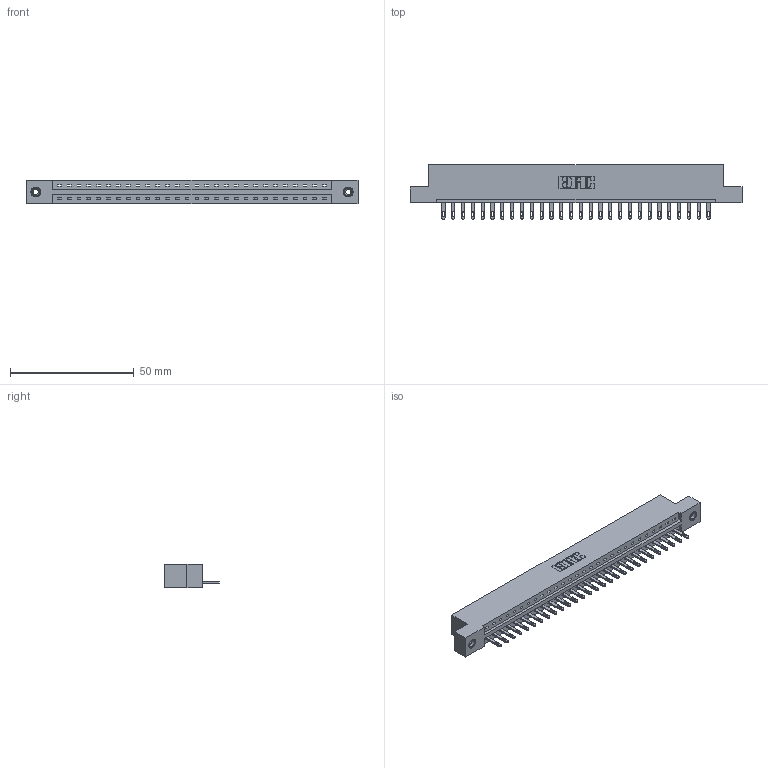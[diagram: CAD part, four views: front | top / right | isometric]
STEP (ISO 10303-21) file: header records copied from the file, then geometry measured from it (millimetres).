
FILE_DESCRIPTION (( 'STEP AP203' ), '1' );
FILE_NAME ('337-028-500-108.STEP', '2018-08-06T08:46:16', ( '' ), ( '' ), 'SwSTEP 2.0', 'SolidWorks 2016', '' );
FILE_SCHEMA (( 'CONFIG_CONTROL_DESIGN' ));
Length unit declared in the file: inch
Products named in the file (4): 337 Part_Flush Mounting Lugs - 0.156 Dia-TI; 345-292-001_345-293-100; 345-250-001_345-250-003-102; 337-028-500-108
Assembly tree (31 placements, depth 2):
  337-028-500-108
    337 Part_Flush Mounting Lugs - 0.156 Dia-TI
    345-292-001_345-293-100  x28
    345-250-001_345-250-003-102  x2
Bounding box: 133.96 x 21.85 x 9.4 mm (x, y, z)
Volume: 13758.5 mm3; surface area: 14234.7 mm2
Topology: 31 solids, 31 shells, 1798 faces, 5487 edges, 3650 vertices
Faces by surface type: plane 1222, cylinder 560, cone 12, torus 4
Entity records: 23740 total; most frequent: CARTESIAN_POINT 4113, ORIENTED_EDGE 4070, DIRECTION 3525, EDGE_CURVE 2035, VECTOR 1883, LINE 1883, VERTEX_POINT 1352, AXIS2_PLACEMENT_3D 821
